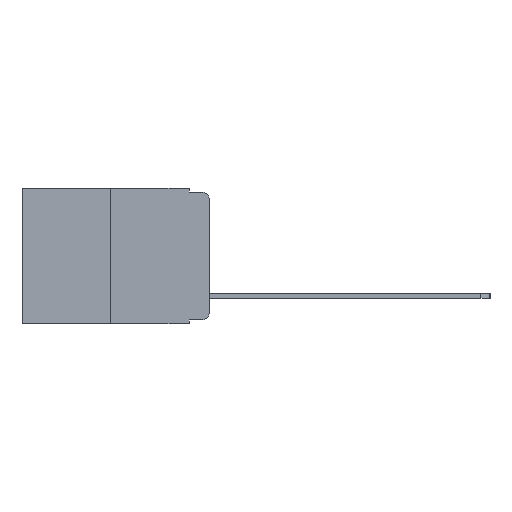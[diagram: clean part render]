
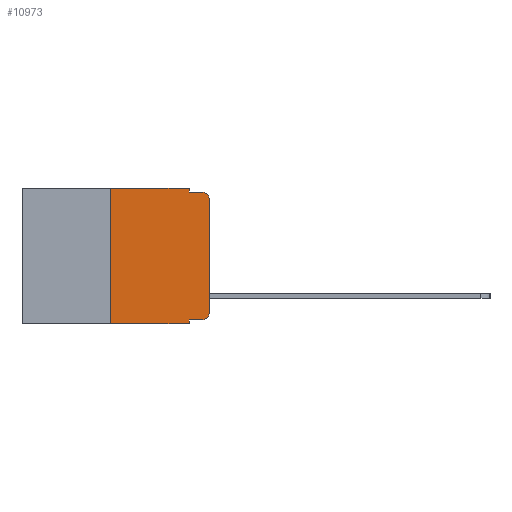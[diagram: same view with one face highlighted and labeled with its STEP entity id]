
A CAD part, left-side view. The second image highlights one B-rep face of the part: STEP entity #10973.
In plain terms, the highlighted planar face has unit normal (-1, 0, 0).
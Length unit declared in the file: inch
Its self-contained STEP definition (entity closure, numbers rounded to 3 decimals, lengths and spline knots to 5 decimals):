
#29 = VERTEX_POINT ( 'NONE', #5617 ) ;
#240 = LINE ( 'NONE', #15572, #3666 ) ;
#569 = AXIS2_PLACEMENT_3D ( 'NONE', #3151, #13182, #4637 ) ;
#593 = CARTESIAN_POINT ( 'NONE',  ( 0., 0.473, -0.343 ) ) ;
#603 = VERTEX_POINT ( 'NONE', #11754 ) ;
#745 = DIRECTION ( 'NONE',  ( 0., 0., 1. ) ) ;
#930 = CARTESIAN_POINT ( 'NONE',  ( 0., 0., -0.313 ) ) ;
#946 = EDGE_CURVE ( 'NONE', #603, #18004, #18094, .T. ) ;
#1887 = EDGE_CURVE ( 'NONE', #3615, #8133, #13108, .T. ) ;
#2103 = EDGE_CURVE ( 'NONE', #603, #18298, #2180, .T. ) ;
#2180 = LINE ( 'NONE', #17250, #17264 ) ;
#2226 = CARTESIAN_POINT ( 'NONE',  ( 0., 0.25, 0. ) ) ;
#2897 = CARTESIAN_POINT ( 'NONE',  ( 0., 0.051, 0. ) ) ;
#2901 = LINE ( 'NONE', #2226, #17397 ) ;
#3151 = CARTESIAN_POINT ( 'NONE',  ( 0., 0.02, -0.313 ) ) ;
#3226 = EDGE_CURVE ( 'NONE', #7131, #3615, #2901, .T. ) ;
#3615 = VERTEX_POINT ( 'NONE', #15066 ) ;
#3666 = VECTOR ( 'NONE', #7156, 39.37008 ) ;
#4209 = EDGE_CURVE ( 'NONE', #8133, #29, #6506, .T. ) ;
#4478 = FACE_OUTER_BOUND ( 'NONE', #14527, .T. ) ;
#4637 = DIRECTION ( 'NONE',  ( 0., 0., -1. ) ) ;
#5150 = EDGE_CURVE ( 'NONE', #29, #7682, #240, .T. ) ;
#5195 = ORIENTED_EDGE ( 'NONE', *, *, #16435, .T. ) ;
#5567 = CARTESIAN_POINT ( 'NONE',  ( 0., 0., 0. ) ) ;
#5617 = CARTESIAN_POINT ( 'NONE',  ( 0., 0.051, -0.01 ) ) ;
#5653 = ORIENTED_EDGE ( 'NONE', *, *, #946, .T. ) ;
#5811 = CARTESIAN_POINT ( 'NONE',  ( 0., 0.02, -0.03 ) ) ;
#6189 = DIRECTION ( 'NONE',  ( 0., -1., 0. ) ) ;
#6240 = CARTESIAN_POINT ( 'NONE',  ( 0., 0.051, -0.333 ) ) ;
#6324 = ORIENTED_EDGE ( 'NONE', *, *, #18156, .T. ) ;
#6506 = LINE ( 'NONE', #12806, #13642 ) ;
#6682 = AXIS2_PLACEMENT_3D ( 'NONE', #5811, #15678, #7285 ) ;
#7090 = EDGE_CURVE ( 'NONE', #7803, #7682, #9999, .T. ) ;
#7131 = VERTEX_POINT ( 'NONE', #8930 ) ;
#7156 = DIRECTION ( 'NONE',  ( 0., -1., 0. ) ) ;
#7285 = DIRECTION ( 'NONE',  ( 0., 0., -1. ) ) ;
#7682 = VERTEX_POINT ( 'NONE', #17241 ) ;
#7803 = VERTEX_POINT ( 'NONE', #13511 ) ;
#8133 = VERTEX_POINT ( 'NONE', #2897 ) ;
#8188 = ORIENTED_EDGE ( 'NONE', *, *, #3226, .F. ) ;
#8930 = CARTESIAN_POINT ( 'NONE',  ( 0., 0.25, -0.343 ) ) ;
#8950 = PLANE ( 'NONE',  #16535 ) ;
#9860 = VECTOR ( 'NONE', #10111, 39.37008 ) ;
#9999 = CIRCLE ( 'NONE', #6682, 0.02 ) ;
#10022 = ORIENTED_EDGE ( 'NONE', *, *, #18485, .T. ) ;
#10111 = DIRECTION ( 'NONE',  ( 0., -1., 0. ) ) ;
#10360 = VECTOR ( 'NONE', #14087, 39.37008 ) ;
#10382 = DIRECTION ( 'NONE',  ( 0., 0., -1. ) ) ;
#10659 = ORIENTED_EDGE ( 'NONE', *, *, #7090, .T. ) ;
#10973 = ADVANCED_FACE ( 'NONE', ( #4478 ), #8950, .F. ) ;
#11754 = CARTESIAN_POINT ( 'NONE',  ( 0., 0.051, -0.333 ) ) ;
#12522 = DIRECTION ( 'NONE',  ( 0., -1., 0. ) ) ;
#12806 = CARTESIAN_POINT ( 'NONE',  ( 0., 0.051, 0. ) ) ;
#12820 = ORIENTED_EDGE ( 'NONE', *, *, #2103, .F. ) ;
#12848 = DIRECTION ( 'NONE',  ( 0., 0., -1. ) ) ;
#13108 = LINE ( 'NONE', #14554, #9860 ) ;
#13182 = DIRECTION ( 'NONE',  ( -1., 0., 0. ) ) ;
#13442 = VECTOR ( 'NONE', #12522, 39.37008 ) ;
#13511 = CARTESIAN_POINT ( 'NONE',  ( 0., 0., -0.03 ) ) ;
#13642 = VECTOR ( 'NONE', #12848, 39.37008 ) ;
#14000 = LINE ( 'NONE', #5567, #10360 ) ;
#14087 = DIRECTION ( 'NONE',  ( 0., 0., 1. ) ) ;
#14527 = EDGE_LOOP ( 'NONE', ( #6324, #10659, #17799, #18203, #18594, #8188, #5195, #12820, #5653, #10022 ) ) ;
#14554 = CARTESIAN_POINT ( 'NONE',  ( 0., 0.473, 0. ) ) ;
#14654 = VECTOR ( 'NONE', #6189, 39.37008 ) ;
#15066 = CARTESIAN_POINT ( 'NONE',  ( 0., 0.25, 0. ) ) ;
#15493 = CARTESIAN_POINT ( 'NONE',  ( 0., 0.051, -0.343 ) ) ;
#15572 = CARTESIAN_POINT ( 'NONE',  ( 0., 0.051, -0.01 ) ) ;
#15678 = DIRECTION ( 'NONE',  ( -1., 0., 0. ) ) ;
#15812 = CARTESIAN_POINT ( 'NONE',  ( 0., 0.473, 0. ) ) ;
#16435 = EDGE_CURVE ( 'NONE', #7131, #18298, #16985, .T. ) ;
#16535 = AXIS2_PLACEMENT_3D ( 'NONE', #15812, #18389, #10382 ) ;
#16900 = CIRCLE ( 'NONE', #569, 0.02 ) ;
#16985 = LINE ( 'NONE', #593, #13442 ) ;
#17241 = CARTESIAN_POINT ( 'NONE',  ( 0., 0.02, -0.01 ) ) ;
#17250 = CARTESIAN_POINT ( 'NONE',  ( 0., 0.051, 0. ) ) ;
#17264 = VECTOR ( 'NONE', #17287, 39.37008 ) ;
#17287 = DIRECTION ( 'NONE',  ( 0., 0., -1. ) ) ;
#17397 = VECTOR ( 'NONE', #745, 39.37008 ) ;
#17714 = CARTESIAN_POINT ( 'NONE',  ( 0., 0.02, -0.333 ) ) ;
#17799 = ORIENTED_EDGE ( 'NONE', *, *, #5150, .F. ) ;
#18004 = VERTEX_POINT ( 'NONE', #17714 ) ;
#18094 = LINE ( 'NONE', #6240, #14654 ) ;
#18156 = EDGE_CURVE ( 'NONE', #18242, #7803, #14000, .T. ) ;
#18203 = ORIENTED_EDGE ( 'NONE', *, *, #4209, .F. ) ;
#18242 = VERTEX_POINT ( 'NONE', #930 ) ;
#18298 = VERTEX_POINT ( 'NONE', #15493 ) ;
#18389 = DIRECTION ( 'NONE',  ( 1., 0., 0. ) ) ;
#18485 = EDGE_CURVE ( 'NONE', #18004, #18242, #16900, .T. ) ;
#18594 = ORIENTED_EDGE ( 'NONE', *, *, #1887, .F. ) ;
